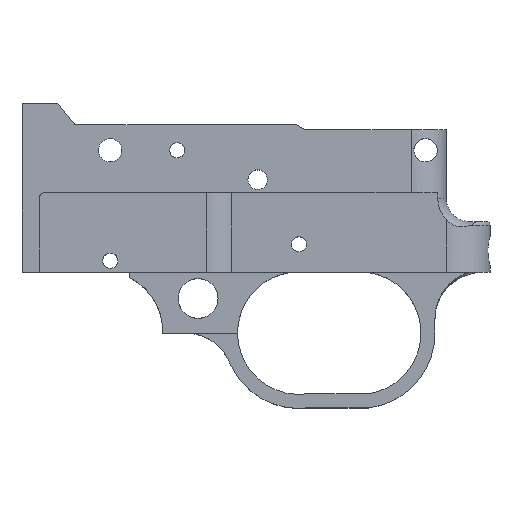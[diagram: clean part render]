
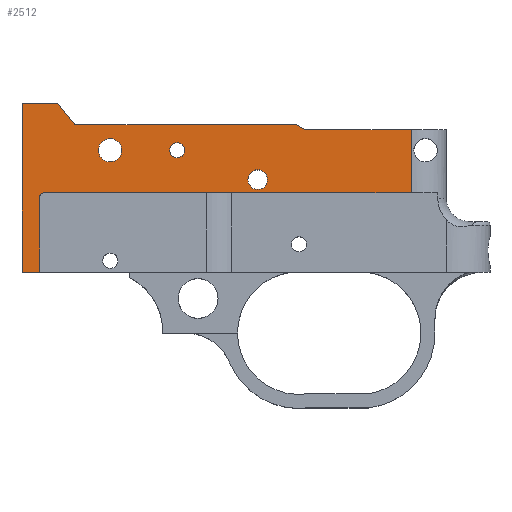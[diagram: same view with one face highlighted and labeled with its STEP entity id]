
A CAD part, top view. The second image highlights one B-rep face of the part: STEP entity #2512.
In plain terms, the highlighted planar face has unit normal (0, 0, 1).
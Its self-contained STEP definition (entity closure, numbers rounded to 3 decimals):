
#11 = DIRECTION ( 'NONE',  ( 1., 0., 0. ) ) ;
#78 = DIRECTION ( 'NONE',  ( -1., 0., 0. ) ) ;
#118 = AXIS2_PLACEMENT_3D ( 'NONE', #1814, #147, #1090 ) ;
#147 = DIRECTION ( 'NONE',  ( 0., 0., -1. ) ) ;
#243 = CARTESIAN_POINT ( 'NONE',  ( -68.11, 26.1, 30.327 ) ) ;
#250 = EDGE_CURVE ( 'NONE', #892, #3836, #4462, .T. ) ;
#275 = EDGE_CURVE ( 'NONE', #3606, #510, #4997, .T. ) ;
#332 = DIRECTION ( 'NONE',  ( 0., -1., 0. ) ) ;
#341 = CARTESIAN_POINT ( 'NONE',  ( -54.635, 26.1, 30.327 ) ) ;
#355 = EDGE_CURVE ( 'NONE', #1550, #3836, #2857, .T. ) ;
#444 = VERTEX_POINT ( 'NONE', #842 ) ;
#463 = CARTESIAN_POINT ( 'NONE',  ( -78.14, 31.5, 30.327 ) ) ;
#465 = EDGE_CURVE ( 'NONE', #510, #3606, #532, .T. ) ;
#480 = CARTESIAN_POINT ( 'NONE',  ( -85.69, 17., 30.327 ) ) ;
#510 = VERTEX_POINT ( 'NONE', #2342 ) ;
#522 = CARTESIAN_POINT ( 'NONE',  ( -84.69, 16., 30.327 ) ) ;
#532 = CIRCLE ( 'NONE', #2140, 2.1 ) ;
#538 = EDGE_CURVE ( 'NONE', #892, #949, #3159, .T. ) ;
#552 = AXIS2_PLACEMENT_3D ( 'NONE', #3732, #1424, #4110 ) ;
#630 = FACE_BOUND ( 'NONE', #783, .T. ) ;
#637 = EDGE_CURVE ( 'NONE', #444, #2283, #4694, .T. ) ;
#729 = EDGE_CURVE ( 'NONE', #4432, #2283, #1523, .T. ) ;
#755 = ORIENTED_EDGE ( 'NONE', *, *, #2082, .T. ) ;
#757 = CARTESIAN_POINT ( 'NONE',  ( -28.74, 30.5, 30.327 ) ) ;
#783 = EDGE_LOOP ( 'NONE', ( #3717, #3969 ) ) ;
#800 = VERTEX_POINT ( 'NONE', #3126 ) ;
#812 = CARTESIAN_POINT ( 'NONE',  ( -81.84, 36.08, 30.327 ) ) ;
#842 = CARTESIAN_POINT ( 'NONE',  ( -89.44, 36.08, 30.327 ) ) ;
#892 = VERTEX_POINT ( 'NONE', #4644 ) ;
#906 = VECTOR ( 'NONE', #332, 1000. ) ;
#912 = DIRECTION ( 'NONE',  ( 0., 0., 1. ) ) ;
#949 = VERTEX_POINT ( 'NONE', #4938 ) ;
#1008 = VECTOR ( 'NONE', #11, 1000. ) ;
#1036 = LINE ( 'NONE', #4586, #2849 ) ;
#1052 = EDGE_CURVE ( 'NONE', #800, #949, #5052, .T. ) ;
#1090 = DIRECTION ( 'NONE',  ( -1., 0., 0. ) ) ;
#1127 = ORIENTED_EDGE ( 'NONE', *, *, #637, .F. ) ;
#1305 = CIRCLE ( 'NONE', #552, 2.5 ) ;
#1355 = EDGE_CURVE ( 'NONE', #444, #800, #1937, .T. ) ;
#1376 = EDGE_CURVE ( 'NONE', #4189, #3180, #1036, .T. ) ;
#1416 = EDGE_CURVE ( 'NONE', #1651, #4016, #1812, .T. ) ;
#1424 = DIRECTION ( 'NONE',  ( 0., 0., 1. ) ) ;
#1465 = EDGE_CURVE ( 'NONE', #3180, #3633, #1573, .T. ) ;
#1489 = EDGE_LOOP ( 'NONE', ( #4045, #1882 ) ) ;
#1523 = LINE ( 'NONE', #1902, #4456 ) ;
#1528 = DIRECTION ( 'NONE',  ( 0.894, -0.447, 0. ) ) ;
#1531 = CARTESIAN_POINT ( 'NONE',  ( -57.885, 26.1, 30.327 ) ) ;
#1542 = CARTESIAN_POINT ( 'NONE',  ( -89.44, 31.5, 30.327 ) ) ;
#1550 = VERTEX_POINT ( 'NONE', #2127 ) ;
#1560 = FACE_BOUND ( 'NONE', #1489, .T. ) ;
#1573 = LINE ( 'NONE', #3783, #4509 ) ;
#1593 = DIRECTION ( 'NONE',  ( 1., 0., 0. ) ) ;
#1651 = VERTEX_POINT ( 'NONE', #1531 ) ;
#1810 = CARTESIAN_POINT ( 'NONE',  ( -6.24, 30.5, 30.327 ) ) ;
#1812 = CIRCLE ( 'NONE', #4411, 1.625 ) ;
#1814 = CARTESIAN_POINT ( 'NONE',  ( -89.44, 31.5, 30.327 ) ) ;
#1860 = DIRECTION ( 'NONE',  ( 1., 0., 0. ) ) ;
#1882 = ORIENTED_EDGE ( 'NONE', *, *, #2914, .F. ) ;
#1902 = CARTESIAN_POINT ( 'NONE',  ( -81.84, 36.08, 30.327 ) ) ;
#1937 = LINE ( 'NONE', #1542, #906 ) ;
#1989 = VERTEX_POINT ( 'NONE', #3648 ) ;
#2004 = VECTOR ( 'NONE', #3667, 1000. ) ;
#2038 = LINE ( 'NONE', #4287, #1008 ) ;
#2071 = DIRECTION ( 'NONE',  ( 0., 0., 1. ) ) ;
#2082 = EDGE_CURVE ( 'NONE', #1550, #3633, #4926, .T. ) ;
#2127 = CARTESIAN_POINT ( 'NONE',  ( -6.24, 17., 30.327 ) ) ;
#2140 = AXIS2_PLACEMENT_3D ( 'NONE', #4652, #4272, #1593 ) ;
#2178 = ORIENTED_EDGE ( 'NONE', *, *, #729, .T. ) ;
#2183 = ORIENTED_EDGE ( 'NONE', *, *, #3372, .F. ) ;
#2261 = CARTESIAN_POINT ( 'NONE',  ( -89.44, 36.08, 30.327 ) ) ;
#2283 = VERTEX_POINT ( 'NONE', #812 ) ;
#2342 = CARTESIAN_POINT ( 'NONE',  ( -36.94, 19.8, 30.327 ) ) ;
#2494 = ORIENTED_EDGE ( 'NONE', *, *, #1052, .T. ) ;
#2499 = AXIS2_PLACEMENT_3D ( 'NONE', #4353, #2071, #4735 ) ;
#2507 = EDGE_LOOP ( 'NONE', ( #4797, #755, #2622, #2535, #2183, #2178, #1127, #3198, #2494, #3829, #3074 ) ) ;
#2512 = ADVANCED_FACE ( 'NONE', ( #3492, #630, #1560, #4497 ), #4774, .F. ) ;
#2535 = ORIENTED_EDGE ( 'NONE', *, *, #1376, .F. ) ;
#2622 = ORIENTED_EDGE ( 'NONE', *, *, #1465, .F. ) ;
#2661 = CARTESIAN_POINT ( 'NONE',  ( -6.24, 31.5, 30.327 ) ) ;
#2674 = DIRECTION ( 'NONE',  ( 0., 1., 0. ) ) ;
#2675 = VECTOR ( 'NONE', #3412, 1000. ) ;
#2685 = AXIS2_PLACEMENT_3D ( 'NONE', #2868, #2890, #2913 ) ;
#2800 = CARTESIAN_POINT ( 'NONE',  ( -84.69, 17., 30.327 ) ) ;
#2836 = EDGE_LOOP ( 'NONE', ( #4094, #2918 ) ) ;
#2849 = VECTOR ( 'NONE', #1528, 1000. ) ;
#2857 = LINE ( 'NONE', #480, #3756 ) ;
#2868 = CARTESIAN_POINT ( 'NONE',  ( -70.61, 26.1, 30.327 ) ) ;
#2890 = DIRECTION ( 'NONE',  ( 0., 0., 1. ) ) ;
#2913 = DIRECTION ( 'NONE',  ( 1., 0., 0. ) ) ;
#2914 = EDGE_CURVE ( 'NONE', #1989, #3204, #4969, .T. ) ;
#2918 = ORIENTED_EDGE ( 'NONE', *, *, #275, .F. ) ;
#3018 = DIRECTION ( 'NONE',  ( 1., 0., 0. ) ) ;
#3074 = ORIENTED_EDGE ( 'NONE', *, *, #250, .T. ) ;
#3126 = CARTESIAN_POINT ( 'NONE',  ( -89.44, 0., 30.327 ) ) ;
#3159 = LINE ( 'NONE', #3466, #4162 ) ;
#3180 = VERTEX_POINT ( 'NONE', #757 ) ;
#3198 = ORIENTED_EDGE ( 'NONE', *, *, #1355, .T. ) ;
#3204 = VERTEX_POINT ( 'NONE', #243 ) ;
#3230 = DIRECTION ( 'NONE',  ( 1., 0., 0. ) ) ;
#3252 = DIRECTION ( 'NONE',  ( 0., 0., -1. ) ) ;
#3280 = CARTESIAN_POINT ( 'NONE',  ( -89.44, 0., 30.327 ) ) ;
#3372 = EDGE_CURVE ( 'NONE', #4432, #4189, #2038, .T. ) ;
#3412 = DIRECTION ( 'NONE',  ( 1., 0., 0. ) ) ;
#3452 = EDGE_CURVE ( 'NONE', #4016, #1651, #3838, .T. ) ;
#3466 = CARTESIAN_POINT ( 'NONE',  ( -85.69, 0., 30.327 ) ) ;
#3492 = FACE_BOUND ( 'NONE', #2836, .T. ) ;
#3606 = VERTEX_POINT ( 'NONE', #3716 ) ;
#3612 = EDGE_CURVE ( 'NONE', #3204, #1989, #1305, .T. ) ;
#3615 = CARTESIAN_POINT ( 'NONE',  ( -39.04, 19.8, 30.327 ) ) ;
#3633 = VERTEX_POINT ( 'NONE', #1810 ) ;
#3648 = CARTESIAN_POINT ( 'NONE',  ( -73.11, 26.1, 30.327 ) ) ;
#3667 = DIRECTION ( 'NONE',  ( 1., 0., 0. ) ) ;
#3716 = CARTESIAN_POINT ( 'NONE',  ( -41.14, 19.8, 30.327 ) ) ;
#3717 = ORIENTED_EDGE ( 'NONE', *, *, #3452, .F. ) ;
#3732 = CARTESIAN_POINT ( 'NONE',  ( -70.61, 26.1, 30.327 ) ) ;
#3756 = VECTOR ( 'NONE', #4340, 1000. ) ;
#3783 = CARTESIAN_POINT ( 'NONE',  ( 1.26, 30.5, 30.327 ) ) ;
#3829 = ORIENTED_EDGE ( 'NONE', *, *, #538, .F. ) ;
#3836 = VERTEX_POINT ( 'NONE', #2800 ) ;
#3838 = CIRCLE ( 'NONE', #2499, 1.625 ) ;
#3855 = DIRECTION ( 'NONE',  ( 0., -1., 0. ) ) ;
#3953 = CARTESIAN_POINT ( 'NONE',  ( -30.74, 31.5, 30.327 ) ) ;
#3969 = ORIENTED_EDGE ( 'NONE', *, *, #1416, .F. ) ;
#4016 = VERTEX_POINT ( 'NONE', #341 ) ;
#4040 = VECTOR ( 'NONE', #2674, 1000. ) ;
#4045 = ORIENTED_EDGE ( 'NONE', *, *, #3612, .F. ) ;
#4094 = ORIENTED_EDGE ( 'NONE', *, *, #465, .F. ) ;
#4110 = DIRECTION ( 'NONE',  ( 1., 0., 0. ) ) ;
#4162 = VECTOR ( 'NONE', #3855, 1000. ) ;
#4189 = VERTEX_POINT ( 'NONE', #3953 ) ;
#4272 = DIRECTION ( 'NONE',  ( 0., 0., 1. ) ) ;
#4287 = CARTESIAN_POINT ( 'NONE',  ( -89.44, 31.5, 30.327 ) ) ;
#4340 = DIRECTION ( 'NONE',  ( -1., 0., 0. ) ) ;
#4353 = CARTESIAN_POINT ( 'NONE',  ( -56.26, 26.1, 30.327 ) ) ;
#4411 = AXIS2_PLACEMENT_3D ( 'NONE', #4927, #4536, #1860 ) ;
#4432 = VERTEX_POINT ( 'NONE', #463 ) ;
#4456 = VECTOR ( 'NONE', #4568, 1000. ) ;
#4462 = CIRCLE ( 'NONE', #4529, 1. ) ;
#4497 = FACE_OUTER_BOUND ( 'NONE', #2507, .T. ) ;
#4509 = VECTOR ( 'NONE', #3018, 1000. ) ;
#4529 = AXIS2_PLACEMENT_3D ( 'NONE', #522, #3252, #78 ) ;
#4536 = DIRECTION ( 'NONE',  ( 0., 0., 1. ) ) ;
#4568 = DIRECTION ( 'NONE',  ( -0.628, 0.778, 0. ) ) ;
#4586 = CARTESIAN_POINT ( 'NONE',  ( -30.74, 31.5, 30.327 ) ) ;
#4644 = CARTESIAN_POINT ( 'NONE',  ( -85.69, 16., 30.327 ) ) ;
#4652 = CARTESIAN_POINT ( 'NONE',  ( -39.04, 19.8, 30.327 ) ) ;
#4694 = LINE ( 'NONE', #2261, #2675 ) ;
#4735 = DIRECTION ( 'NONE',  ( 1., 0., 0. ) ) ;
#4774 = PLANE ( 'NONE',  #118 ) ;
#4797 = ORIENTED_EDGE ( 'NONE', *, *, #355, .F. ) ;
#4926 = LINE ( 'NONE', #2661, #4040 ) ;
#4927 = CARTESIAN_POINT ( 'NONE',  ( -56.26, 26.1, 30.327 ) ) ;
#4938 = CARTESIAN_POINT ( 'NONE',  ( -85.69, 0., 30.327 ) ) ;
#4969 = CIRCLE ( 'NONE', #2685, 2.5 ) ;
#4997 = CIRCLE ( 'NONE', #5042, 2.1 ) ;
#5042 = AXIS2_PLACEMENT_3D ( 'NONE', #3615, #912, #3230 ) ;
#5052 = LINE ( 'NONE', #3280, #2004 ) ;
